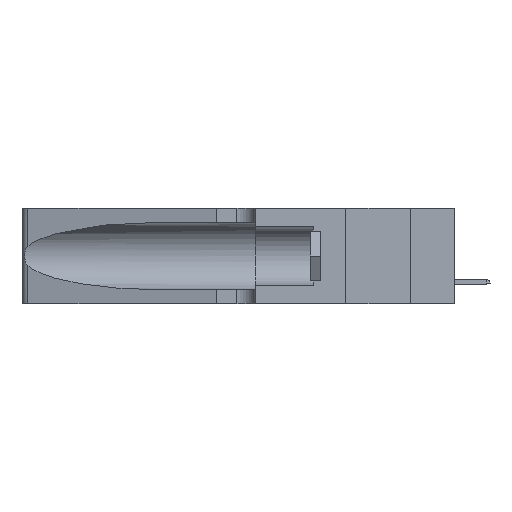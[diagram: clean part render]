
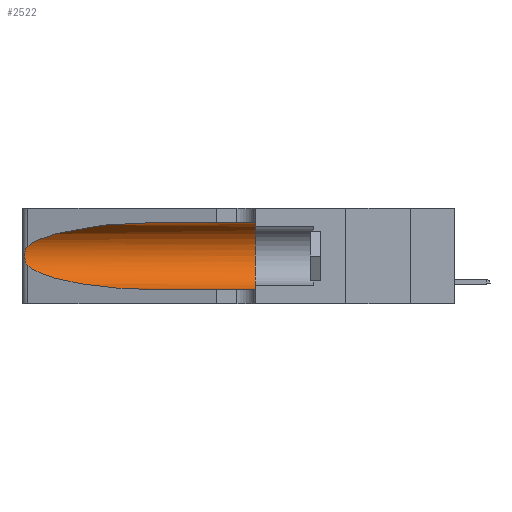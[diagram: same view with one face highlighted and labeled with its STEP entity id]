
A CAD part, left-side view. The second image highlights one B-rep face of the part: STEP entity #2522.
In plain terms, the highlighted cylindrical face has radius 3.308 mm (diameter 6.617 mm), a partial arc.
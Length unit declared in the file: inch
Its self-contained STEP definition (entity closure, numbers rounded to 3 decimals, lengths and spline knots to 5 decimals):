
#236 = CARTESIAN_POINT ( 'NONE',  ( 0.1305, 0.35, 0.185 ) ) ;
#1247 = VECTOR ( 'NONE', #2676, 39.37008 ) ;
#1308 = ORIENTED_EDGE ( 'NONE', *, *, #21937, .F. ) ;
#1521 = CARTESIAN_POINT ( 'NONE',  ( 0.1305, 0.35, 0.31525 ) ) ;
#1987 =( BOUNDED_CURVE ( )  B_SPLINE_CURVE ( 3, ( #13834, #13958, #21419, #11535 ),
 .UNSPECIFIED., .F., .T. ) 
 B_SPLINE_CURVE_WITH_KNOTS ( ( 4, 4 ),
 ( 1.5708, 2.84003 ),
 .UNSPECIFIED. ) 
 CURVE ( )  GEOMETRIC_REPRESENTATION_ITEM ( )  RATIONAL_B_SPLINE_CURVE ( ( 1., 0.87, 0.87, 1. ) ) 
 REPRESENTATION_ITEM ( '' )  );
#2430 = LINE ( 'NONE', #19431, #1247 ) ;
#2522 = ADVANCED_FACE ( 'NONE', ( #16032 ), #14093, .F. ) ;
#2676 = DIRECTION ( 'NONE',  ( 0., -1., 0. ) ) ;
#3473 = VERTEX_POINT ( 'NONE', #9930 ) ;
#3498 = CARTESIAN_POINT ( 'NONE',  ( 0.25639, 1.23186, 0.15144 ) ) ;
#4709 = CARTESIAN_POINT ( 'NONE',  ( 0.25487, 1.22718, 0.22369 ) ) ;
#5217 = CARTESIAN_POINT ( 'NONE',  ( 0.26018, 1.23835, 0.19895 ) ) ;
#5812 = CARTESIAN_POINT ( 'NONE',  ( 0.18966, 0.96281, 0.05475 ) ) ;
#6419 = DIRECTION ( 'NONE',  ( 0., 0., -1. ) ) ;
#6709 = DIRECTION ( 'NONE',  ( 0., -1., 0. ) ) ;
#6811 = VERTEX_POINT ( 'NONE', #20589 ) ;
#6831 = CARTESIAN_POINT ( 'NONE',  ( 0.26017, 1.23833, 0.17102 ) ) ;
#7175 = CARTESIAN_POINT ( 'NONE',  ( 0.25856, 1.23593, 0.16098 ) ) ;
#7460 = ORIENTED_EDGE ( 'NONE', *, *, #19074, .T. ) ;
#8012 = CARTESIAN_POINT ( 'NONE',  ( 0.25487, 1.22718, 0.14631 ) ) ;
#8206 = EDGE_CURVE ( 'NONE', #3473, #23273, #17576, .T. ) ;
#9201 = DIRECTION ( 'NONE',  ( 0., 1., 0. ) ) ;
#9313 = AXIS2_PLACEMENT_3D ( 'NONE', #10077, #15908, #6419 ) ;
#9547 = AXIS2_PLACEMENT_3D ( 'NONE', #236, #9201, #15043 ) ;
#9930 = CARTESIAN_POINT ( 'NONE',  ( 0.1305, 0.72297, 0.05475 ) ) ;
#10077 = CARTESIAN_POINT ( 'NONE',  ( 0.1305, 1.61858, 0.185 ) ) ;
#10885 = EDGE_CURVE ( 'NONE', #18617, #23273, #20880, .T. ) ;
#10952 = CARTESIAN_POINT ( 'NONE',  ( 0.25555, 1.22993, 0.14849 ) ) ;
#11352 = EDGE_CURVE ( 'NONE', #6811, #20961, #1987, .T. ) ;
#11535 = CARTESIAN_POINT ( 'NONE',  ( 0.25487, 1.22718, 0.22369 ) ) ;
#11977 = CARTESIAN_POINT ( 'NONE',  ( 0.1305, 1.61858, 0.05475 ) ) ;
#12709 = EDGE_LOOP ( 'NONE', ( #17765, #7460, #24072, #18370, #13464, #1308 ) ) ;
#12711 = VERTEX_POINT ( 'NONE', #8012 ) ;
#13249 = CARTESIAN_POINT ( 'NONE',  ( 0.1305, 0.72297, 0.05475 ) ) ;
#13464 = ORIENTED_EDGE ( 'NONE', *, *, #10885, .F. ) ;
#13834 = CARTESIAN_POINT ( 'NONE',  ( 0.1305, 0.72297, 0.31525 ) ) ;
#13958 = CARTESIAN_POINT ( 'NONE',  ( 0.18966, 0.96281, 0.31525 ) ) ;
#14093 = CYLINDRICAL_SURFACE ( 'NONE', #9313, 0.13025 ) ;
#14480 = CARTESIAN_POINT ( 'NONE',  ( 0.25639, 1.23184, 0.21858 ) ) ;
#14590 = CARTESIAN_POINT ( 'NONE',  ( 0.25487, 1.22718, 0.22369 ) ) ;
#15043 = DIRECTION ( 'NONE',  ( 0., 0., 1. ) ) ;
#15253 = EDGE_CURVE ( 'NONE', #12711, #3473, #21227, .T. ) ;
#15908 = DIRECTION ( 'NONE',  ( 0., -1., 0. ) ) ;
#16032 = FACE_OUTER_BOUND ( 'NONE', #12709, .T. ) ;
#16207 = CARTESIAN_POINT ( 'NONE',  ( 0.25555, 1.22994, 0.2215 ) ) ;
#16444 = CARTESIAN_POINT ( 'NONE',  ( 0.25854, 1.2359, 0.20912 ) ) ;
#17153 = CARTESIAN_POINT ( 'NONE',  ( 0.25487, 1.22718, 0.14631 ) ) ;
#17183 = CARTESIAN_POINT ( 'NONE',  ( 0.25487, 1.22718, 0.14631 ) ) ;
#17576 = LINE ( 'NONE', #11977, #18446 ) ;
#17765 = ORIENTED_EDGE ( 'NONE', *, *, #11352, .T. ) ;
#18370 = ORIENTED_EDGE ( 'NONE', *, *, #8206, .T. ) ;
#18446 = VECTOR ( 'NONE', #6709, 39.37008 ) ;
#18617 = VERTEX_POINT ( 'NONE', #1521 ) ;
#19074 = EDGE_CURVE ( 'NONE', #20961, #12711, #21687, .T. ) ;
#19431 = CARTESIAN_POINT ( 'NONE',  ( 0.1305, 1.61858, 0.31525 ) ) ;
#19662 = CARTESIAN_POINT ( 'NONE',  ( 0.1305, 0.35, 0.05475 ) ) ;
#20589 = CARTESIAN_POINT ( 'NONE',  ( 0.1305, 0.72297, 0.31525 ) ) ;
#20880 = CIRCLE ( 'NONE', #9547, 0.13025 ) ;
#20961 = VERTEX_POINT ( 'NONE', #4709 ) ;
#21227 =( BOUNDED_CURVE ( )  B_SPLINE_CURVE ( 3, ( #17153, #22541, #5812, #13249 ),
 .UNSPECIFIED., .F., .T. ) 
 B_SPLINE_CURVE_WITH_KNOTS ( ( 4, 4 ),
 ( 3.44316, 4.71239 ),
 .UNSPECIFIED. ) 
 CURVE ( )  GEOMETRIC_REPRESENTATION_ITEM ( )  RATIONAL_B_SPLINE_CURVE ( ( 1., 0.87, 0.87, 1. ) ) 
 REPRESENTATION_ITEM ( '' )  );
#21419 = CARTESIAN_POINT ( 'NONE',  ( 0.2373, 1.15595, 0.28018 ) ) ;
#21687 = B_SPLINE_CURVE_WITH_KNOTS ( 'NONE', 3,
 ( #14590, #16207, #14480, #21958, #16444, #5217, #23555, #23915, #6831, #7175, #22071, #3498, #10952, #17183 ),
 .UNSPECIFIED., .F., .F.,
 ( 4, 2, 2, 2, 2, 2, 4 ),
 ( 0., 0.00027, 0.00053, 0.00107, 0.0016, 0.00187, 0.00214 ),
 .UNSPECIFIED. ) ;
#21937 = EDGE_CURVE ( 'NONE', #6811, #18617, #2430, .T. ) ;
#21958 = CARTESIAN_POINT ( 'NONE',  ( 0.25787, 1.23484, 0.2124 ) ) ;
#22071 = CARTESIAN_POINT ( 'NONE',  ( 0.25789, 1.23486, 0.15765 ) ) ;
#22541 = CARTESIAN_POINT ( 'NONE',  ( 0.2373, 1.15595, 0.08982 ) ) ;
#23273 = VERTEX_POINT ( 'NONE', #19662 ) ;
#23555 = CARTESIAN_POINT ( 'NONE',  ( 0.26075, 1.23896, 0.19203 ) ) ;
#23915 = CARTESIAN_POINT ( 'NONE',  ( 0.26075, 1.23896, 0.178 ) ) ;
#24072 = ORIENTED_EDGE ( 'NONE', *, *, #15253, .T. ) ;
